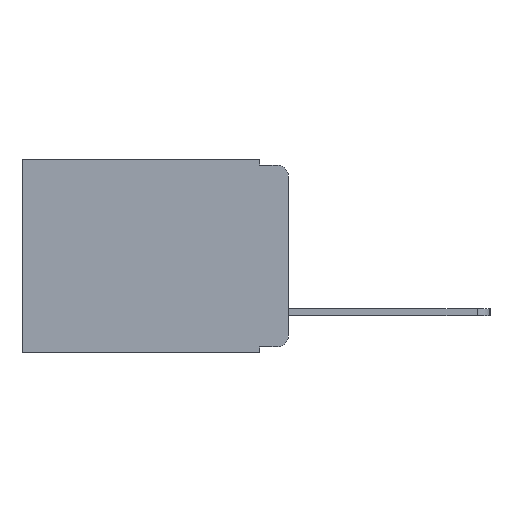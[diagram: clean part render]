
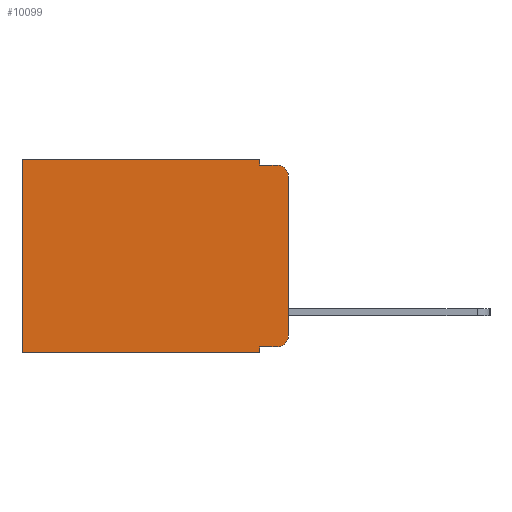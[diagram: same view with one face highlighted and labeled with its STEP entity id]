
A CAD part, left-side view. The second image highlights one B-rep face of the part: STEP entity #10099.
In plain terms, the highlighted planar face has unit normal (-1, 0, 0).
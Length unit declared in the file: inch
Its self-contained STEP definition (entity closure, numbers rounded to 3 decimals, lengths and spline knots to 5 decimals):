
#106 = ORIENTED_EDGE ( 'NONE', *, *, #8463, .F. ) ;
#271 = LINE ( 'NONE', #8298, #6961 ) ;
#1012 = VERTEX_POINT ( 'NONE', #8915 ) ;
#1067 = ORIENTED_EDGE ( 'NONE', *, *, #5108, .T. ) ;
#1196 = CIRCLE ( 'NONE', #8165, 0.02 ) ;
#1254 = DIRECTION ( 'NONE',  ( 0., 1., 0. ) ) ;
#1284 = LINE ( 'NONE', #6101, #3993 ) ;
#1548 = VERTEX_POINT ( 'NONE', #8602 ) ;
#1556 = EDGE_CURVE ( 'NONE', #2929, #3562, #1284, .T. ) ;
#1749 = CARTESIAN_POINT ( 'NONE',  ( 0.298, 0., 0. ) ) ;
#2165 = EDGE_CURVE ( 'NONE', #2929, #8967, #7810, .T. ) ;
#2345 = DIRECTION ( 'NONE',  ( 0., -1., 0. ) ) ;
#2614 = ORIENTED_EDGE ( 'NONE', *, *, #2165, .T. ) ;
#2643 = CARTESIAN_POINT ( 'NONE',  ( 0.298, 0.051, 0. ) ) ;
#2885 = ORIENTED_EDGE ( 'NONE', *, *, #5783, .T. ) ;
#2929 = VERTEX_POINT ( 'NONE', #9885 ) ;
#2967 = VECTOR ( 'NONE', #11066, 39.37008 ) ;
#3043 = ORIENTED_EDGE ( 'NONE', *, *, #1556, .F. ) ;
#3313 = EDGE_CURVE ( 'NONE', #1012, #6258, #7376, .T. ) ;
#3324 = ORIENTED_EDGE ( 'NONE', *, *, #3370, .F. ) ;
#3370 = EDGE_CURVE ( 'NONE', #3562, #3630, #10960, .T. ) ;
#3394 = LINE ( 'NONE', #11062, #9943 ) ;
#3562 = VERTEX_POINT ( 'NONE', #5928 ) ;
#3574 = ORIENTED_EDGE ( 'NONE', *, *, #8065, .T. ) ;
#3630 = VERTEX_POINT ( 'NONE', #8523 ) ;
#3723 = VERTEX_POINT ( 'NONE', #3907 ) ;
#3742 = ORIENTED_EDGE ( 'NONE', *, *, #6842, .T. ) ;
#3889 = ORIENTED_EDGE ( 'NONE', *, *, #9019, .F. ) ;
#3907 = CARTESIAN_POINT ( 'NONE',  ( 0.298, 0.051, -0.01 ) ) ;
#3954 = VECTOR ( 'NONE', #1254, 39.37008 ) ;
#3993 = VECTOR ( 'NONE', #10130, 39.37008 ) ;
#4019 = ORIENTED_EDGE ( 'NONE', *, *, #3313, .F. ) ;
#4137 = VECTOR ( 'NONE', #9687, 39.37008 ) ;
#4294 = CARTESIAN_POINT ( 'NONE',  ( 0.298, 0.051, -0.333 ) ) ;
#4583 = CARTESIAN_POINT ( 'NONE',  ( 0.298, 0., 0. ) ) ;
#4637 = CARTESIAN_POINT ( 'NONE',  ( 0.298, 0.02, -0.01 ) ) ;
#4800 = CARTESIAN_POINT ( 'NONE',  ( 0.298, 0.02, -0.333 ) ) ;
#5016 = FACE_OUTER_BOUND ( 'NONE', #7450, .T. ) ;
#5108 = EDGE_CURVE ( 'NONE', #1012, #7930, #1196, .T. ) ;
#5383 = DIRECTION ( 'NONE',  ( 1., 0., 0. ) ) ;
#5527 = VECTOR ( 'NONE', #2345, 39.37008 ) ;
#5783 = EDGE_CURVE ( 'NONE', #8967, #6258, #8476, .T. ) ;
#5863 = AXIS2_PLACEMENT_3D ( 'NONE', #1749, #5383, #11191 ) ;
#5928 = CARTESIAN_POINT ( 'NONE',  ( 0.298, 0.051, -0.343 ) ) ;
#6101 = CARTESIAN_POINT ( 'NONE',  ( 0.298, 0.051, 0. ) ) ;
#6258 = VERTEX_POINT ( 'NONE', #8797 ) ;
#6407 = AXIS2_PLACEMENT_3D ( 'NONE', #11197, #6430, #6419 ) ;
#6419 = DIRECTION ( 'NONE',  ( 0., 0., -1. ) ) ;
#6430 = DIRECTION ( 'NONE',  ( -1., 0., 0. ) ) ;
#6772 = LINE ( 'NONE', #4583, #4137 ) ;
#6842 = EDGE_CURVE ( 'NONE', #10400, #1548, #6772, .T. ) ;
#6961 = VECTOR ( 'NONE', #9130, 39.37008 ) ;
#7053 = CARTESIAN_POINT ( 'NONE',  ( 0.298, 0., 0. ) ) ;
#7376 = LINE ( 'NONE', #7053, #2967 ) ;
#7420 = CARTESIAN_POINT ( 'NONE',  ( 0.298, 0.473, 0. ) ) ;
#7450 = EDGE_LOOP ( 'NONE', ( #4019, #1067, #106, #3889, #3742, #3574, #3324, #3043, #2614, #2885 ) ) ;
#7810 = LINE ( 'NONE', #4294, #5527 ) ;
#7930 = VERTEX_POINT ( 'NONE', #4637 ) ;
#8065 = EDGE_CURVE ( 'NONE', #1548, #3630, #11327, .T. ) ;
#8165 = AXIS2_PLACEMENT_3D ( 'NONE', #9729, #9267, #9643 ) ;
#8249 = DIRECTION ( 'NONE',  ( 0., 0., -1. ) ) ;
#8298 = CARTESIAN_POINT ( 'NONE',  ( 0.298, 0.051, 0. ) ) ;
#8463 = EDGE_CURVE ( 'NONE', #3723, #7930, #3394, .T. ) ;
#8476 = CIRCLE ( 'NONE', #6407, 0.02 ) ;
#8523 = CARTESIAN_POINT ( 'NONE',  ( 0.298, 0.473, -0.343 ) ) ;
#8602 = CARTESIAN_POINT ( 'NONE',  ( 0.298, 0.473, 0. ) ) ;
#8746 = PLANE ( 'NONE',  #5863 ) ;
#8797 = CARTESIAN_POINT ( 'NONE',  ( 0.298, 0., -0.313 ) ) ;
#8915 = CARTESIAN_POINT ( 'NONE',  ( 0.298, 0., -0.03 ) ) ;
#8967 = VERTEX_POINT ( 'NONE', #4800 ) ;
#9019 = EDGE_CURVE ( 'NONE', #10400, #3723, #271, .T. ) ;
#9130 = DIRECTION ( 'NONE',  ( 0., 0., -1. ) ) ;
#9193 = VECTOR ( 'NONE', #8249, 39.37008 ) ;
#9267 = DIRECTION ( 'NONE',  ( -1., 0., 0. ) ) ;
#9643 = DIRECTION ( 'NONE',  ( 0., 0., -1. ) ) ;
#9687 = DIRECTION ( 'NONE',  ( 0., 1., 0. ) ) ;
#9729 = CARTESIAN_POINT ( 'NONE',  ( 0.298, 0.02, -0.03 ) ) ;
#9885 = CARTESIAN_POINT ( 'NONE',  ( 0.298, 0.051, -0.333 ) ) ;
#9943 = VECTOR ( 'NONE', #10245, 39.37008 ) ;
#9956 = CARTESIAN_POINT ( 'NONE',  ( 0.298, 0., -0.343 ) ) ;
#10099 = ADVANCED_FACE ( 'NONE', ( #5016 ), #8746, .F. ) ;
#10130 = DIRECTION ( 'NONE',  ( 0., 0., -1. ) ) ;
#10245 = DIRECTION ( 'NONE',  ( 0., -1., 0. ) ) ;
#10400 = VERTEX_POINT ( 'NONE', #2643 ) ;
#10960 = LINE ( 'NONE', #9956, #3954 ) ;
#11062 = CARTESIAN_POINT ( 'NONE',  ( 0.298, 0.051, -0.01 ) ) ;
#11066 = DIRECTION ( 'NONE',  ( 0., 0., -1. ) ) ;
#11191 = DIRECTION ( 'NONE',  ( 0., 0., -1. ) ) ;
#11197 = CARTESIAN_POINT ( 'NONE',  ( 0.298, 0.02, -0.313 ) ) ;
#11327 = LINE ( 'NONE', #7420, #9193 ) ;
